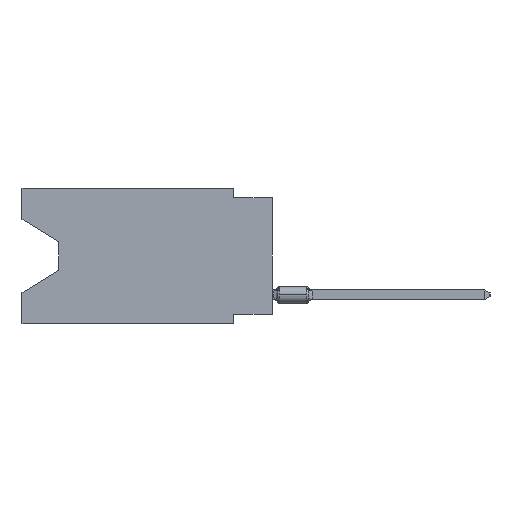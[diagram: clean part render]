
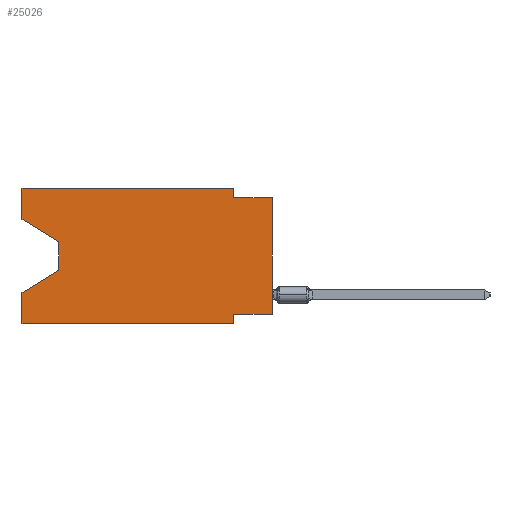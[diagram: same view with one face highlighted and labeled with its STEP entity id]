
A CAD part, left-side view. The second image highlights one B-rep face of the part: STEP entity #25026.
In plain terms, the highlighted planar face has unit normal (-1, 0, 0).
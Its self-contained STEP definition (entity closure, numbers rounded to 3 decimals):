
#855 = DIRECTION ( 'NONE',  ( 0., 0., -1. ) ) ;
#1012 = LINE ( 'NONE', #28997, #28719 ) ;
#1249 = ORIENTED_EDGE ( 'NONE', *, *, #27830, .F. ) ;
#1861 = VERTEX_POINT ( 'NONE', #34856 ) ;
#2184 = VERTEX_POINT ( 'NONE', #3248 ) ;
#2301 = VERTEX_POINT ( 'NONE', #7246 ) ;
#2403 = ORIENTED_EDGE ( 'NONE', *, *, #34616, .T. ) ;
#2832 = DIRECTION ( 'NONE',  ( 0., 0., -1. ) ) ;
#2952 = DIRECTION ( 'NONE',  ( 0., 0., 1. ) ) ;
#2999 = EDGE_CURVE ( 'NONE', #23546, #31482, #22265, .T. ) ;
#3093 = ORIENTED_EDGE ( 'NONE', *, *, #16315, .T. ) ;
#3248 = CARTESIAN_POINT ( 'NONE',  ( 0., 13.97, -3.505 ) ) ;
#3743 = DIRECTION ( 'NONE',  ( 0., 0., 1. ) ) ;
#3759 = CARTESIAN_POINT ( 'NONE',  ( 0., 16.383, -2.038 ) ) ;
#3881 = PLANE ( 'NONE',  #27703 ) ;
#4074 = FACE_OUTER_BOUND ( 'NONE', #13192, .T. ) ;
#4324 = VERTEX_POINT ( 'NONE', #6094 ) ;
#4833 = DIRECTION ( 'NONE',  ( 0., 0., 1. ) ) ;
#5051 = LINE ( 'NONE', #30429, #8883 ) ;
#5061 = EDGE_CURVE ( 'NONE', #2301, #18398, #17325, .T. ) ;
#5195 = VECTOR ( 'NONE', #8273, 1000. ) ;
#5551 = EDGE_CURVE ( 'NONE', #31482, #4324, #11820, .T. ) ;
#5952 = CARTESIAN_POINT ( 'NONE',  ( 0., 0., -0.635 ) ) ;
#6094 = CARTESIAN_POINT ( 'NONE',  ( 0., 2.54, 0. ) ) ;
#6347 = LINE ( 'NONE', #5952, #24335 ) ;
#6714 = CARTESIAN_POINT ( 'NONE',  ( 0., 13.97, -3.505 ) ) ;
#7246 = CARTESIAN_POINT ( 'NONE',  ( 0., 13.97, -5.385 ) ) ;
#7526 = CARTESIAN_POINT ( 'NONE',  ( 0., 2.54, -0.635 ) ) ;
#8066 = CARTESIAN_POINT ( 'NONE',  ( 0., 16.383, -8.89 ) ) ;
#8273 = DIRECTION ( 'NONE',  ( 0., -1., 0. ) ) ;
#8883 = VECTOR ( 'NONE', #2832, 1000. ) ;
#9000 = DIRECTION ( 'NONE',  ( 0., 0., -1. ) ) ;
#9164 = DIRECTION ( 'NONE',  ( 0., -1., 0. ) ) ;
#10077 = VERTEX_POINT ( 'NONE', #30473 ) ;
#10484 = DIRECTION ( 'NONE',  ( 1., 0., 0. ) ) ;
#11157 = VERTEX_POINT ( 'NONE', #14452 ) ;
#11815 = CARTESIAN_POINT ( 'NONE',  ( 0., 0., -8.255 ) ) ;
#11820 = LINE ( 'NONE', #17480, #30839 ) ;
#12025 = LINE ( 'NONE', #33156, #14973 ) ;
#13192 = EDGE_LOOP ( 'NONE', ( #3093, #29743, #20126, #29746, #2403, #20463, #28581, #25509, #22060, #1249, #25900, #37995 ) ) ;
#14452 = CARTESIAN_POINT ( 'NONE',  ( 0., 2.54, -8.255 ) ) ;
#14973 = VECTOR ( 'NONE', #9000, 1000. ) ;
#15528 = VECTOR ( 'NONE', #2952, 1000. ) ;
#15794 = DIRECTION ( 'NONE',  ( 0., 0., -1. ) ) ;
#15994 = LINE ( 'NONE', #6714, #38413 ) ;
#16315 = EDGE_CURVE ( 'NONE', #23546, #2184, #17186, .T. ) ;
#16765 = CARTESIAN_POINT ( 'NONE',  ( 0., 16.383, 0. ) ) ;
#17186 = LINE ( 'NONE', #3759, #33214 ) ;
#17325 = LINE ( 'NONE', #19537, #23054 ) ;
#17369 = LINE ( 'NONE', #8066, #5195 ) ;
#17480 = CARTESIAN_POINT ( 'NONE',  ( 0., 16.383, 0. ) ) ;
#17719 = CARTESIAN_POINT ( 'NONE',  ( 0., 0., -0.635 ) ) ;
#18078 = DIRECTION ( 'NONE',  ( 0., -1., 0. ) ) ;
#18398 = VERTEX_POINT ( 'NONE', #22848 ) ;
#19537 = CARTESIAN_POINT ( 'NONE',  ( 0., 13.97, -5.385 ) ) ;
#19779 = LINE ( 'NONE', #29041, #32632 ) ;
#20126 = ORIENTED_EDGE ( 'NONE', *, *, #5061, .T. ) ;
#20463 = ORIENTED_EDGE ( 'NONE', *, *, #32262, .F. ) ;
#20640 = EDGE_CURVE ( 'NONE', #1861, #18398, #21465, .T. ) ;
#21465 = LINE ( 'NONE', #27707, #15528 ) ;
#21742 = VECTOR ( 'NONE', #3743, 1000. ) ;
#22060 = ORIENTED_EDGE ( 'NONE', *, *, #22521, .F. ) ;
#22265 = LINE ( 'NONE', #31336, #21742 ) ;
#22521 = EDGE_CURVE ( 'NONE', #22669, #39307, #6347, .T. ) ;
#22669 = VERTEX_POINT ( 'NONE', #7526 ) ;
#22848 = CARTESIAN_POINT ( 'NONE',  ( 0., 16.383, -6.852 ) ) ;
#23054 = VECTOR ( 'NONE', #35212, 1000. ) ;
#23546 = VERTEX_POINT ( 'NONE', #33333 ) ;
#24335 = VECTOR ( 'NONE', #9164, 1000. ) ;
#24505 = DIRECTION ( 'NONE',  ( 0., -0.855, -0.519 ) ) ;
#25026 = ADVANCED_FACE ( 'NONE', ( #4074 ), #3881, .F. ) ;
#25509 = ORIENTED_EDGE ( 'NONE', *, *, #37429, .T. ) ;
#25900 = ORIENTED_EDGE ( 'NONE', *, *, #5551, .F. ) ;
#26532 = CARTESIAN_POINT ( 'NONE',  ( 0., 16.383, 0. ) ) ;
#27703 = AXIS2_PLACEMENT_3D ( 'NONE', #16765, #10484, #855 ) ;
#27707 = CARTESIAN_POINT ( 'NONE',  ( 0., 16.383, 0. ) ) ;
#27830 = EDGE_CURVE ( 'NONE', #4324, #22669, #12025, .T. ) ;
#28362 = VERTEX_POINT ( 'NONE', #11815 ) ;
#28581 = ORIENTED_EDGE ( 'NONE', *, *, #29715, .F. ) ;
#28719 = VECTOR ( 'NONE', #4833, 1000. ) ;
#28997 = CARTESIAN_POINT ( 'NONE',  ( 0., 0., 0. ) ) ;
#29041 = CARTESIAN_POINT ( 'NONE',  ( 0., 0., -8.255 ) ) ;
#29715 = EDGE_CURVE ( 'NONE', #28362, #11157, #19779, .T. ) ;
#29743 = ORIENTED_EDGE ( 'NONE', *, *, #38581, .T. ) ;
#29746 = ORIENTED_EDGE ( 'NONE', *, *, #20640, .F. ) ;
#30429 = CARTESIAN_POINT ( 'NONE',  ( 0., 2.54, -8.89 ) ) ;
#30473 = CARTESIAN_POINT ( 'NONE',  ( 0., 2.54, -8.89 ) ) ;
#30839 = VECTOR ( 'NONE', #18078, 1000. ) ;
#31336 = CARTESIAN_POINT ( 'NONE',  ( 0., 16.383, 0. ) ) ;
#31482 = VERTEX_POINT ( 'NONE', #26532 ) ;
#32262 = EDGE_CURVE ( 'NONE', #11157, #10077, #5051, .T. ) ;
#32632 = VECTOR ( 'NONE', #35654, 1000. ) ;
#33156 = CARTESIAN_POINT ( 'NONE',  ( 0., 2.54, 0. ) ) ;
#33214 = VECTOR ( 'NONE', #24505, 1000. ) ;
#33333 = CARTESIAN_POINT ( 'NONE',  ( 0., 16.383, -2.038 ) ) ;
#34616 = EDGE_CURVE ( 'NONE', #1861, #10077, #17369, .T. ) ;
#34856 = CARTESIAN_POINT ( 'NONE',  ( 0., 16.383, -8.89 ) ) ;
#35212 = DIRECTION ( 'NONE',  ( 0., 0.855, -0.519 ) ) ;
#35654 = DIRECTION ( 'NONE',  ( 0., 1., 0. ) ) ;
#37429 = EDGE_CURVE ( 'NONE', #28362, #39307, #1012, .T. ) ;
#37995 = ORIENTED_EDGE ( 'NONE', *, *, #2999, .F. ) ;
#38413 = VECTOR ( 'NONE', #15794, 1000. ) ;
#38581 = EDGE_CURVE ( 'NONE', #2184, #2301, #15994, .T. ) ;
#39307 = VERTEX_POINT ( 'NONE', #17719 ) ;
